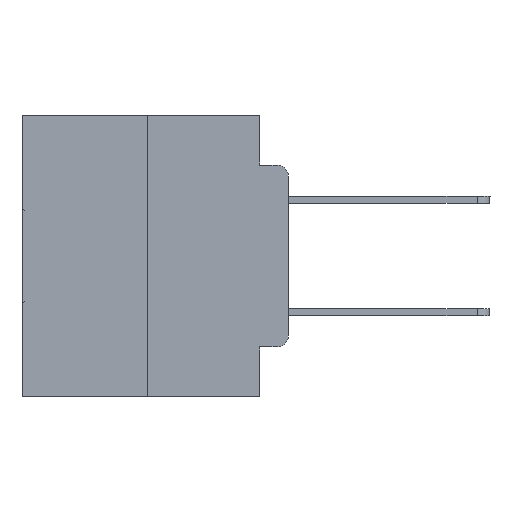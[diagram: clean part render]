
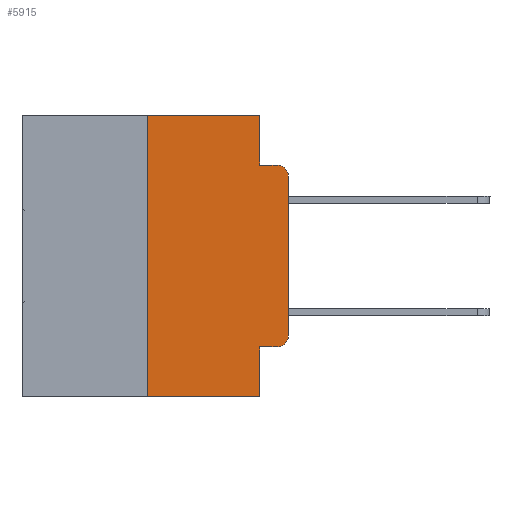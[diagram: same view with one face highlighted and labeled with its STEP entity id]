
A CAD part, left-side view. The second image highlights one B-rep face of the part: STEP entity #5915.
In plain terms, the highlighted planar face has unit normal (-1, 0, 0).
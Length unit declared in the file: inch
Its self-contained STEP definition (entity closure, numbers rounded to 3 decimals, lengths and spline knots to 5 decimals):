
#585 = EDGE_CURVE ( 'NONE', #27120, #17484, #23280, .T. ) ;
#864 = VECTOR ( 'NONE', #12576, 39.37008 ) ;
#877 = PLANE ( 'NONE',  #27923 ) ;
#885 = DIRECTION ( 'NONE',  ( 0., 0., -1. ) ) ;
#1203 = CIRCLE ( 'NONE', #30989, 0.02 ) ;
#1282 = VERTEX_POINT ( 'NONE', #19007 ) ;
#1396 = EDGE_CURVE ( 'NONE', #1282, #27120, #27727, .T. ) ;
#1502 = LINE ( 'NONE', #13041, #7974 ) ;
#1560 = CARTESIAN_POINT ( 'NONE',  ( 0., 0.051, -0.5 ) ) ;
#2020 = VECTOR ( 'NONE', #25462, 39.37008 ) ;
#2767 = VERTEX_POINT ( 'NONE', #12517 ) ;
#3232 = CARTESIAN_POINT ( 'NONE',  ( 0., 0.02, -0.1085 ) ) ;
#3475 = ORIENTED_EDGE ( 'NONE', *, *, #1396, .F. ) ;
#3861 = VERTEX_POINT ( 'NONE', #26398 ) ;
#4050 = VECTOR ( 'NONE', #12165, 39.37008 ) ;
#4790 = EDGE_CURVE ( 'NONE', #1282, #27110, #5903, .T. ) ;
#4864 = CARTESIAN_POINT ( 'NONE',  ( 0., 0., -0.1085 ) ) ;
#5166 = VECTOR ( 'NONE', #13828, 39.37008 ) ;
#5687 = DIRECTION ( 'NONE',  ( 0., 0., -1. ) ) ;
#5903 = LINE ( 'NONE', #6518, #5166 ) ;
#5915 = ADVANCED_FACE ( 'NONE', ( #19078 ), #877, .F. ) ;
#6371 = ORIENTED_EDGE ( 'NONE', *, *, #10583, .T. ) ;
#6518 = CARTESIAN_POINT ( 'NONE',  ( 0., 0.473, -0.5 ) ) ;
#6719 = CARTESIAN_POINT ( 'NONE',  ( 0., 0.051, -0.0885 ) ) ;
#6789 = CARTESIAN_POINT ( 'NONE',  ( 0., 0.051, -0.4115 ) ) ;
#7919 = EDGE_CURVE ( 'NONE', #17484, #8793, #1502, .T. ) ;
#7974 = VECTOR ( 'NONE', #885, 39.37008 ) ;
#8739 = LINE ( 'NONE', #6789, #26425 ) ;
#8743 = VERTEX_POINT ( 'NONE', #11416 ) ;
#8793 = VERTEX_POINT ( 'NONE', #6719 ) ;
#9221 = DIRECTION ( 'NONE',  ( 0., -1., 0. ) ) ;
#9978 = CARTESIAN_POINT ( 'NONE',  ( 0., 0.02, -0.3915 ) ) ;
#10122 = CARTESIAN_POINT ( 'NONE',  ( 0., 0.051, -0.0885 ) ) ;
#10379 = VERTEX_POINT ( 'NONE', #4864 ) ;
#10583 = EDGE_CURVE ( 'NONE', #10379, #8743, #25050, .T. ) ;
#10748 = ORIENTED_EDGE ( 'NONE', *, *, #4790, .T. ) ;
#11131 = VECTOR ( 'NONE', #26152, 39.37008 ) ;
#11205 = EDGE_CURVE ( 'NONE', #8793, #8743, #26583, .T. ) ;
#11416 = CARTESIAN_POINT ( 'NONE',  ( 0., 0.02, -0.0885 ) ) ;
#11823 = EDGE_CURVE ( 'NONE', #2767, #20493, #1203, .T. ) ;
#12165 = DIRECTION ( 'NONE',  ( 0., -1., 0. ) ) ;
#12179 = CARTESIAN_POINT ( 'NONE',  ( 0., 0.25, 0. ) ) ;
#12439 = DIRECTION ( 'NONE',  ( 0., 0., -1. ) ) ;
#12517 = CARTESIAN_POINT ( 'NONE',  ( 0., 0.02, -0.4115 ) ) ;
#12576 = DIRECTION ( 'NONE',  ( 0., -1., 0. ) ) ;
#12660 = LINE ( 'NONE', #19052, #11131 ) ;
#13041 = CARTESIAN_POINT ( 'NONE',  ( 0., 0.051, 0. ) ) ;
#13130 = DIRECTION ( 'NONE',  ( 1., 0., 0. ) ) ;
#13420 = EDGE_CURVE ( 'NONE', #3861, #2767, #8739, .T. ) ;
#13828 = DIRECTION ( 'NONE',  ( 0., -1., 0. ) ) ;
#14599 = DIRECTION ( 'NONE',  ( 0., 0., 1. ) ) ;
#14925 = ORIENTED_EDGE ( 'NONE', *, *, #13420, .T. ) ;
#15816 = CARTESIAN_POINT ( 'NONE',  ( 0., 0.051, 0. ) ) ;
#15956 = ORIENTED_EDGE ( 'NONE', *, *, #11205, .F. ) ;
#17079 = EDGE_CURVE ( 'NONE', #20493, #10379, #12660, .T. ) ;
#17484 = VERTEX_POINT ( 'NONE', #27387 ) ;
#18179 = ORIENTED_EDGE ( 'NONE', *, *, #7919, .F. ) ;
#19007 = CARTESIAN_POINT ( 'NONE',  ( 0., 0.25, -0.5 ) ) ;
#19052 = CARTESIAN_POINT ( 'NONE',  ( 0., 0., 0. ) ) ;
#19078 = FACE_OUTER_BOUND ( 'NONE', #29872, .T. ) ;
#20158 = DIRECTION ( 'NONE',  ( -1., 0., 0. ) ) ;
#20493 = VERTEX_POINT ( 'NONE', #27499 ) ;
#21472 = EDGE_CURVE ( 'NONE', #3861, #27110, #26923, .T. ) ;
#23280 = LINE ( 'NONE', #23395, #4050 ) ;
#23318 = CARTESIAN_POINT ( 'NONE',  ( 0., 0.25, 0. ) ) ;
#23395 = CARTESIAN_POINT ( 'NONE',  ( 0., 0.473, 0. ) ) ;
#24923 = ORIENTED_EDGE ( 'NONE', *, *, #585, .F. ) ;
#25050 = CIRCLE ( 'NONE', #26417, 0.02 ) ;
#25462 = DIRECTION ( 'NONE',  ( 0., 0., -1. ) ) ;
#26152 = DIRECTION ( 'NONE',  ( 0., 0., 1. ) ) ;
#26398 = CARTESIAN_POINT ( 'NONE',  ( 0., 0.051, -0.4115 ) ) ;
#26417 = AXIS2_PLACEMENT_3D ( 'NONE', #3232, #20158, #5687 ) ;
#26425 = VECTOR ( 'NONE', #9221, 39.37008 ) ;
#26478 = ORIENTED_EDGE ( 'NONE', *, *, #17079, .T. ) ;
#26583 = LINE ( 'NONE', #10122, #864 ) ;
#26783 = DIRECTION ( 'NONE',  ( -1., 0., 0. ) ) ;
#26923 = LINE ( 'NONE', #15816, #2020 ) ;
#27110 = VERTEX_POINT ( 'NONE', #1560 ) ;
#27120 = VERTEX_POINT ( 'NONE', #23318 ) ;
#27387 = CARTESIAN_POINT ( 'NONE',  ( 0., 0.051, 0. ) ) ;
#27472 = CARTESIAN_POINT ( 'NONE',  ( 0., 0.473, 0. ) ) ;
#27499 = CARTESIAN_POINT ( 'NONE',  ( 0., 0., -0.3915 ) ) ;
#27632 = ORIENTED_EDGE ( 'NONE', *, *, #21472, .F. ) ;
#27663 = ORIENTED_EDGE ( 'NONE', *, *, #11823, .T. ) ;
#27727 = LINE ( 'NONE', #12179, #28480 ) ;
#27923 = AXIS2_PLACEMENT_3D ( 'NONE', #27472, #13130, #29845 ) ;
#28480 = VECTOR ( 'NONE', #14599, 39.37008 ) ;
#29845 = DIRECTION ( 'NONE',  ( 0., 0., -1. ) ) ;
#29872 = EDGE_LOOP ( 'NONE', ( #26478, #6371, #15956, #18179, #24923, #3475, #10748, #27632, #14925, #27663 ) ) ;
#30989 = AXIS2_PLACEMENT_3D ( 'NONE', #9978, #26783, #12439 ) ;
